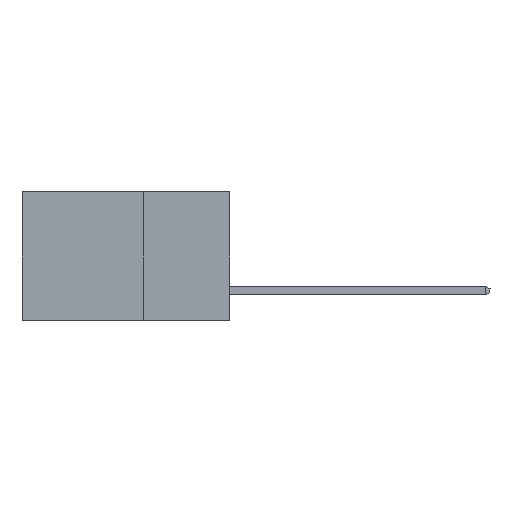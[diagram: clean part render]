
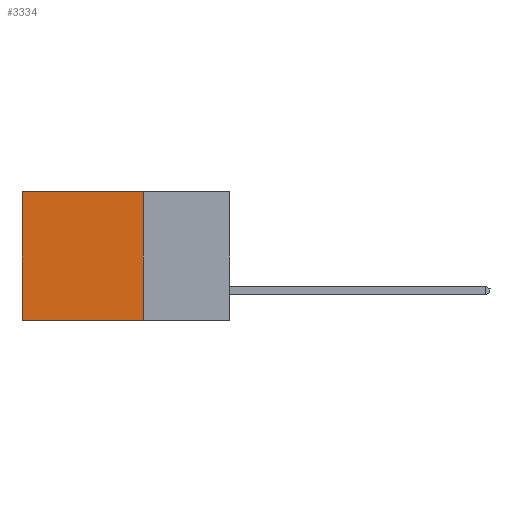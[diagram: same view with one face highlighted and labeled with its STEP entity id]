
A CAD part, left-side view. The second image highlights one B-rep face of the part: STEP entity #3334.
In plain terms, the highlighted planar face has unit normal (-1, 0, 0).
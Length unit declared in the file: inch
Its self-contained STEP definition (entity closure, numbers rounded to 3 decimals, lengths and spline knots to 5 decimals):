
#383 = VECTOR ( 'NONE', #11865, 39.37008 ) ;
#765 = CARTESIAN_POINT ( 'NONE',  ( 0.2615, 0.25, 0. ) ) ;
#1915 = VERTEX_POINT ( 'NONE', #16140 ) ;
#2167 = CARTESIAN_POINT ( 'NONE',  ( 0.2615, 0.25, -0.37 ) ) ;
#2738 = EDGE_CURVE ( 'NONE', #15353, #1915, #15991, .T. ) ;
#3334 = ADVANCED_FACE ( 'NONE', ( #5243 ), #7938, .F. ) ;
#4097 = DIRECTION ( 'NONE',  ( 1., 0., 0. ) ) ;
#4395 = EDGE_LOOP ( 'NONE', ( #11266, #14370, #8206, #5978 ) ) ;
#4402 = VERTEX_POINT ( 'NONE', #11645 ) ;
#5172 = VECTOR ( 'NONE', #7654, 39.37008 ) ;
#5243 = FACE_OUTER_BOUND ( 'NONE', #4395, .T. ) ;
#5262 = DIRECTION ( 'NONE',  ( 0., 1., 0. ) ) ;
#5978 = ORIENTED_EDGE ( 'NONE', *, *, #14333, .T. ) ;
#7654 = DIRECTION ( 'NONE',  ( 0., 1., 0. ) ) ;
#7673 = LINE ( 'NONE', #8259, #383 ) ;
#7938 = PLANE ( 'NONE',  #8827 ) ;
#8206 = ORIENTED_EDGE ( 'NONE', *, *, #14381, .F. ) ;
#8233 = CARTESIAN_POINT ( 'NONE',  ( 0.2615, 0.6, 0. ) ) ;
#8259 = CARTESIAN_POINT ( 'NONE',  ( 0.2615, 0.6, -0.37 ) ) ;
#8288 = CARTESIAN_POINT ( 'NONE',  ( 0.2615, 0.25, -0.37 ) ) ;
#8807 = LINE ( 'NONE', #2167, #16320 ) ;
#8827 = AXIS2_PLACEMENT_3D ( 'NONE', #13262, #4097, #14824 ) ;
#9913 = VERTEX_POINT ( 'NONE', #8233 ) ;
#10645 = EDGE_CURVE ( 'NONE', #9913, #1915, #7673, .T. ) ;
#11266 = ORIENTED_EDGE ( 'NONE', *, *, #10645, .T. ) ;
#11414 = LINE ( 'NONE', #765, #5172 ) ;
#11500 = DIRECTION ( 'NONE',  ( 0., 0., -1. ) ) ;
#11645 = CARTESIAN_POINT ( 'NONE',  ( 0.2615, 0.25, 0. ) ) ;
#11865 = DIRECTION ( 'NONE',  ( 0., 0., -1. ) ) ;
#13262 = CARTESIAN_POINT ( 'NONE',  ( 0.2615, 0.25, -0.37 ) ) ;
#14333 = EDGE_CURVE ( 'NONE', #4402, #9913, #11414, .T. ) ;
#14370 = ORIENTED_EDGE ( 'NONE', *, *, #2738, .F. ) ;
#14381 = EDGE_CURVE ( 'NONE', #4402, #15353, #8807, .T. ) ;
#14824 = DIRECTION ( 'NONE',  ( 0., 0., -1. ) ) ;
#15353 = VERTEX_POINT ( 'NONE', #8288 ) ;
#15991 = LINE ( 'NONE', #17216, #16797 ) ;
#16140 = CARTESIAN_POINT ( 'NONE',  ( 0.2615, 0.6, -0.37 ) ) ;
#16320 = VECTOR ( 'NONE', #11500, 39.37008 ) ;
#16797 = VECTOR ( 'NONE', #5262, 39.37008 ) ;
#17216 = CARTESIAN_POINT ( 'NONE',  ( 0.2615, 0.25, -0.37 ) ) ;
